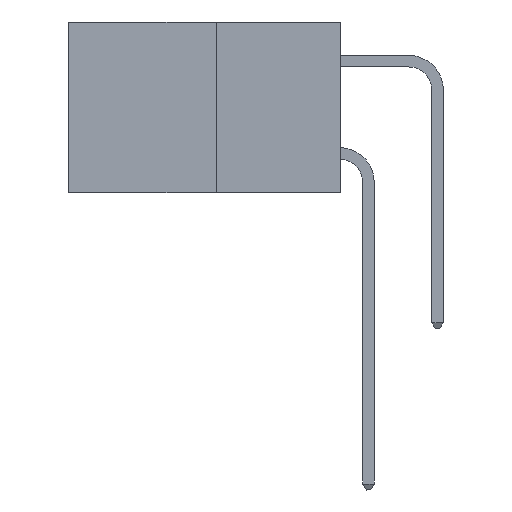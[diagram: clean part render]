
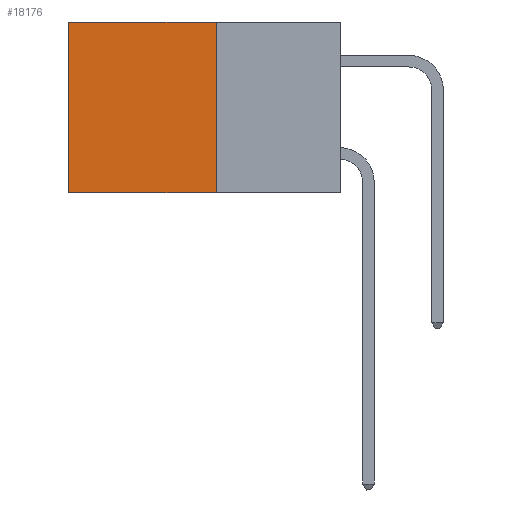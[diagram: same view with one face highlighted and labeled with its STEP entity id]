
A CAD part, left-side view. The second image highlights one B-rep face of the part: STEP entity #18176.
In plain terms, the highlighted planar face has unit normal (-1, 0, 0).
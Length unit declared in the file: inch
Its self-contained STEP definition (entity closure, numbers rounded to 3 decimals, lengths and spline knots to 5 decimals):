
#135 = VERTEX_POINT ( 'NONE', #13247 ) ;
#1201 = DIRECTION ( 'NONE',  ( 0., 1., 0. ) ) ;
#1236 = VERTEX_POINT ( 'NONE', #10248 ) ;
#1262 = VERTEX_POINT ( 'NONE', #8199 ) ;
#1268 = VECTOR ( 'NONE', #20899, 39.37008 ) ;
#2572 = LINE ( 'NONE', #21185, #10904 ) ;
#2908 = DIRECTION ( 'NONE',  ( 0., 1., 0. ) ) ;
#3361 = EDGE_CURVE ( 'NONE', #135, #1236, #10781, .T. ) ;
#4177 = DIRECTION ( 'NONE',  ( 0., 0., -1. ) ) ;
#4225 = VERTEX_POINT ( 'NONE', #17513 ) ;
#5580 = VECTOR ( 'NONE', #19544, 39.37008 ) ;
#6222 = ORIENTED_EDGE ( 'NONE', *, *, #7611, .T. ) ;
#6888 = CARTESIAN_POINT ( 'NONE',  ( 0.277, 0.27, -0.37 ) ) ;
#7262 = EDGE_LOOP ( 'NONE', ( #16342, #15057, #19780, #6222 ) ) ;
#7578 = CARTESIAN_POINT ( 'NONE',  ( 0.277, 0.59, -0.37 ) ) ;
#7611 = EDGE_CURVE ( 'NONE', #4225, #1262, #2572, .T. ) ;
#8199 = CARTESIAN_POINT ( 'NONE',  ( 0.277, 0.59, 0. ) ) ;
#10248 = CARTESIAN_POINT ( 'NONE',  ( 0.277, 0.59, -0.37 ) ) ;
#10781 = LINE ( 'NONE', #6888, #19164 ) ;
#10829 = PLANE ( 'NONE',  #10925 ) ;
#10904 = VECTOR ( 'NONE', #2908, 39.37008 ) ;
#10925 = AXIS2_PLACEMENT_3D ( 'NONE', #12521, #14224, #4177 ) ;
#12521 = CARTESIAN_POINT ( 'NONE',  ( 0.277, 0.27, -0.37 ) ) ;
#12839 = CARTESIAN_POINT ( 'NONE',  ( 0.277, 0.27, -0.37 ) ) ;
#12999 = EDGE_CURVE ( 'NONE', #4225, #135, #19410, .T. ) ;
#13247 = CARTESIAN_POINT ( 'NONE',  ( 0.277, 0.27, -0.37 ) ) ;
#14224 = DIRECTION ( 'NONE',  ( 1., 0., 0. ) ) ;
#15057 = ORIENTED_EDGE ( 'NONE', *, *, #3361, .F. ) ;
#16315 = FACE_OUTER_BOUND ( 'NONE', #7262, .T. ) ;
#16342 = ORIENTED_EDGE ( 'NONE', *, *, #21280, .T. ) ;
#17513 = CARTESIAN_POINT ( 'NONE',  ( 0.277, 0.27, 0. ) ) ;
#18176 = ADVANCED_FACE ( 'NONE', ( #16315 ), #10829, .F. ) ;
#18521 = LINE ( 'NONE', #7578, #1268 ) ;
#19164 = VECTOR ( 'NONE', #1201, 39.37008 ) ;
#19410 = LINE ( 'NONE', #12839, #5580 ) ;
#19544 = DIRECTION ( 'NONE',  ( 0., 0., -1. ) ) ;
#19780 = ORIENTED_EDGE ( 'NONE', *, *, #12999, .F. ) ;
#20899 = DIRECTION ( 'NONE',  ( 0., 0., -1. ) ) ;
#21185 = CARTESIAN_POINT ( 'NONE',  ( 0.277, 0.27, 0. ) ) ;
#21280 = EDGE_CURVE ( 'NONE', #1262, #1236, #18521, .T. ) ;
